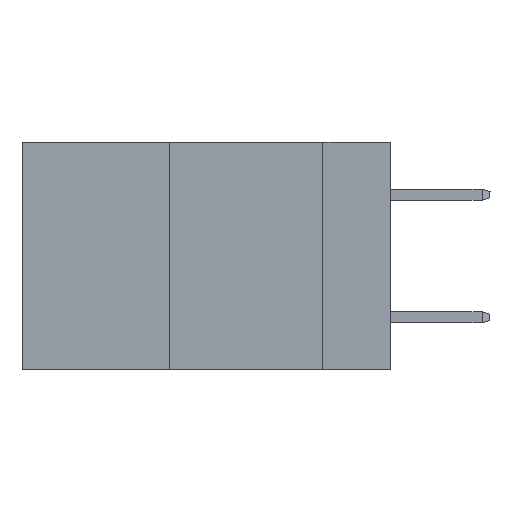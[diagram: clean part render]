
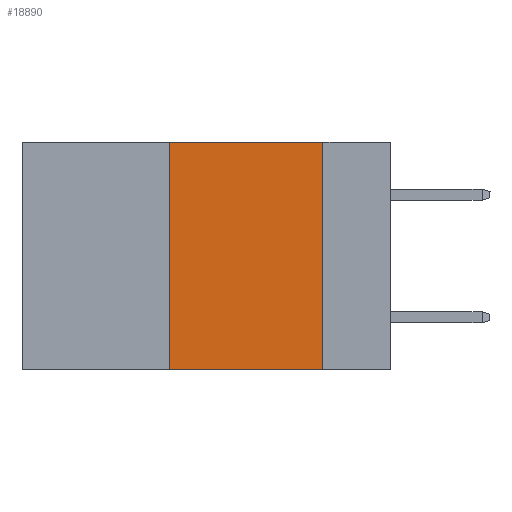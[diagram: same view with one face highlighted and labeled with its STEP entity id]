
A CAD part, left-side view. The second image highlights one B-rep face of the part: STEP entity #18890.
In plain terms, the highlighted planar face has unit normal (-1, 0, 0).
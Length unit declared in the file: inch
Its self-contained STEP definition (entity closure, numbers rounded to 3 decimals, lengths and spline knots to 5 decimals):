
#167 = LINE ( 'NONE', #7107, #2819 ) ;
#220 = CARTESIAN_POINT ( 'NONE',  ( 0., 0.36, -0.37 ) ) ;
#1671 = DIRECTION ( 'NONE',  ( 1., 0., 0. ) ) ;
#2819 = VECTOR ( 'NONE', #20157, 39.37008 ) ;
#2978 = ORIENTED_EDGE ( 'NONE', *, *, #16808, .F. ) ;
#3694 = EDGE_LOOP ( 'NONE', ( #2978, #9034, #9261, #4809 ) ) ;
#4809 = ORIENTED_EDGE ( 'NONE', *, *, #20414, .T. ) ;
#4896 = VECTOR ( 'NONE', #10556, 39.37008 ) ;
#5706 = LINE ( 'NONE', #15764, #12705 ) ;
#5826 = CARTESIAN_POINT ( 'NONE',  ( 0., 0.6, 0. ) ) ;
#6434 = FACE_OUTER_BOUND ( 'NONE', #3694, .T. ) ;
#7035 = CARTESIAN_POINT ( 'NONE',  ( 0., 0.11, -0.37 ) ) ;
#7107 = CARTESIAN_POINT ( 'NONE',  ( 0., 0.11, 0. ) ) ;
#8150 = CARTESIAN_POINT ( 'NONE',  ( 0., 0.6, 0. ) ) ;
#8501 = VERTEX_POINT ( 'NONE', #12080 ) ;
#8845 = LINE ( 'NONE', #5826, #4896 ) ;
#9034 = ORIENTED_EDGE ( 'NONE', *, *, #17177, .F. ) ;
#9261 = ORIENTED_EDGE ( 'NONE', *, *, #12215, .F. ) ;
#10007 = LINE ( 'NONE', #15960, #20859 ) ;
#10475 = VERTEX_POINT ( 'NONE', #10493 ) ;
#10493 = CARTESIAN_POINT ( 'NONE',  ( 0., 0.11, 0. ) ) ;
#10556 = DIRECTION ( 'NONE',  ( 0., -1., 0. ) ) ;
#12080 = CARTESIAN_POINT ( 'NONE',  ( 0., 0.36, 0. ) ) ;
#12215 = EDGE_CURVE ( 'NONE', #20112, #8501, #5706, .T. ) ;
#12705 = VECTOR ( 'NONE', #19174, 39.37008 ) ;
#15764 = CARTESIAN_POINT ( 'NONE',  ( 0., 0.36, 0. ) ) ;
#15960 = CARTESIAN_POINT ( 'NONE',  ( 0., 0.6, -0.37 ) ) ;
#16388 = AXIS2_PLACEMENT_3D ( 'NONE', #8150, #1671, #16499 ) ;
#16499 = DIRECTION ( 'NONE',  ( 0., 0., -1. ) ) ;
#16575 = PLANE ( 'NONE',  #16388 ) ;
#16808 = EDGE_CURVE ( 'NONE', #10475, #19039, #167, .T. ) ;
#17177 = EDGE_CURVE ( 'NONE', #8501, #10475, #8845, .T. ) ;
#17860 = DIRECTION ( 'NONE',  ( 0., -1., 0. ) ) ;
#18890 = ADVANCED_FACE ( 'NONE', ( #6434 ), #16575, .F. ) ;
#19039 = VERTEX_POINT ( 'NONE', #7035 ) ;
#19174 = DIRECTION ( 'NONE',  ( 0., 0., 1. ) ) ;
#20112 = VERTEX_POINT ( 'NONE', #220 ) ;
#20157 = DIRECTION ( 'NONE',  ( 0., 0., -1. ) ) ;
#20414 = EDGE_CURVE ( 'NONE', #20112, #19039, #10007, .T. ) ;
#20859 = VECTOR ( 'NONE', #17860, 39.37008 ) ;
